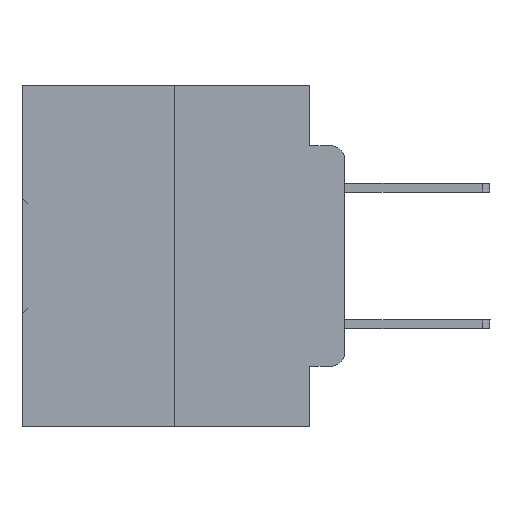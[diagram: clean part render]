
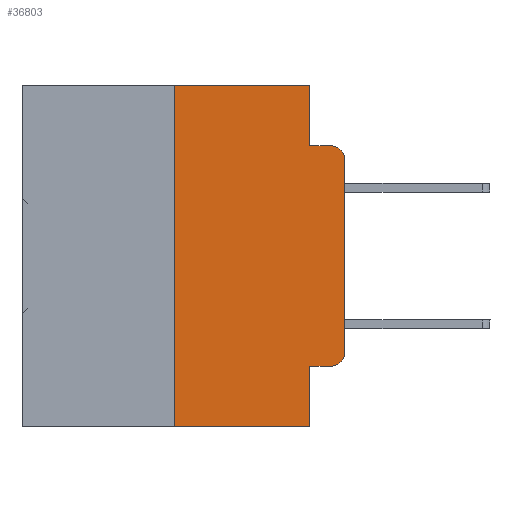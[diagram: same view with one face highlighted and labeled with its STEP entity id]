
A CAD part, left-side view. The second image highlights one B-rep face of the part: STEP entity #36803.
In plain terms, the highlighted planar face has unit normal (-1, 0, 0).
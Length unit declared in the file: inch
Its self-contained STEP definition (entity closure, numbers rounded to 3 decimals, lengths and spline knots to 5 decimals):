
#66 = CARTESIAN_POINT ( 'NONE',  ( 0., 0.02, -0.3915 ) ) ;
#750 = EDGE_CURVE ( 'NONE', #13123, #33339, #28263, .T. ) ;
#777 = VERTEX_POINT ( 'NONE', #26204 ) ;
#805 = ORIENTED_EDGE ( 'NONE', *, *, #27159, .T. ) ;
#1136 = AXIS2_PLACEMENT_3D ( 'NONE', #28376, #11016, #31248 ) ;
#1469 = CARTESIAN_POINT ( 'NONE',  ( 0., 0.051, -0.4115 ) ) ;
#1773 = CIRCLE ( 'NONE', #6889, 0.02 ) ;
#2341 = EDGE_CURVE ( 'NONE', #9298, #10730, #1773, .T. ) ;
#2383 = LINE ( 'NONE', #35653, #30519 ) ;
#2748 = CARTESIAN_POINT ( 'NONE',  ( 0., 0.02, -0.0885 ) ) ;
#4278 = CARTESIAN_POINT ( 'NONE',  ( 0., 0.051, 0. ) ) ;
#4859 = DIRECTION ( 'NONE',  ( 0., 0., 1. ) ) ;
#4932 = ORIENTED_EDGE ( 'NONE', *, *, #24605, .T. ) ;
#5225 = EDGE_CURVE ( 'NONE', #13123, #777, #28075, .T. ) ;
#6889 = AXIS2_PLACEMENT_3D ( 'NONE', #66, #22908, #25892 ) ;
#7152 = DIRECTION ( 'NONE',  ( 0., 0., -1. ) ) ;
#7493 = VECTOR ( 'NONE', #14813, 39.37008 ) ;
#8100 = DIRECTION ( 'NONE',  ( 0., -1., 0. ) ) ;
#8222 = ORIENTED_EDGE ( 'NONE', *, *, #34606, .F. ) ;
#9298 = VERTEX_POINT ( 'NONE', #29091 ) ;
#9443 = EDGE_LOOP ( 'NONE', ( #16734, #4932, #8222, #20383, #10666, #20608, #20315, #22162, #805, #31760 ) ) ;
#10469 = AXIS2_PLACEMENT_3D ( 'NONE', #25110, #33506, #22584 ) ;
#10666 = ORIENTED_EDGE ( 'NONE', *, *, #34669, .F. ) ;
#10730 = VERTEX_POINT ( 'NONE', #23477 ) ;
#10957 = VECTOR ( 'NONE', #28970, 39.37008 ) ;
#11016 = DIRECTION ( 'NONE',  ( 1., 0., 0. ) ) ;
#13123 = VERTEX_POINT ( 'NONE', #31041 ) ;
#13481 = DIRECTION ( 'NONE',  ( 0., -1., 0. ) ) ;
#14813 = DIRECTION ( 'NONE',  ( 0., -1., 0. ) ) ;
#15160 = DIRECTION ( 'NONE',  ( 0., 0., 1. ) ) ;
#15196 = VERTEX_POINT ( 'NONE', #18921 ) ;
#15843 = VECTOR ( 'NONE', #28283, 39.37008 ) ;
#16505 = LINE ( 'NONE', #24801, #18285 ) ;
#16734 = ORIENTED_EDGE ( 'NONE', *, *, #28552, .T. ) ;
#18285 = VECTOR ( 'NONE', #8100, 39.37008 ) ;
#18733 = VECTOR ( 'NONE', #13481, 39.37008 ) ;
#18921 = CARTESIAN_POINT ( 'NONE',  ( 0., 0.051, -0.4115 ) ) ;
#19501 = VERTEX_POINT ( 'NONE', #32627 ) ;
#20314 = CARTESIAN_POINT ( 'NONE',  ( 0., 0.473, -0.5 ) ) ;
#20315 = ORIENTED_EDGE ( 'NONE', *, *, #5225, .T. ) ;
#20383 = ORIENTED_EDGE ( 'NONE', *, *, #35664, .F. ) ;
#20608 = ORIENTED_EDGE ( 'NONE', *, *, #750, .F. ) ;
#21323 = CARTESIAN_POINT ( 'NONE',  ( 0., 0.473, 0. ) ) ;
#21720 = CIRCLE ( 'NONE', #10469, 0.02 ) ;
#22162 = ORIENTED_EDGE ( 'NONE', *, *, #27186, .F. ) ;
#22584 = DIRECTION ( 'NONE',  ( 0., 0., -1. ) ) ;
#22668 = VERTEX_POINT ( 'NONE', #23260 ) ;
#22908 = DIRECTION ( 'NONE',  ( -1., 0., 0. ) ) ;
#23260 = CARTESIAN_POINT ( 'NONE',  ( 0., 0.051, 0. ) ) ;
#23477 = CARTESIAN_POINT ( 'NONE',  ( 0., 0., -0.3915 ) ) ;
#24511 = CARTESIAN_POINT ( 'NONE',  ( 0., 0.25, 0. ) ) ;
#24605 = EDGE_CURVE ( 'NONE', #30196, #31005, #21720, .T. ) ;
#24801 = CARTESIAN_POINT ( 'NONE',  ( 0., 0.051, -0.0885 ) ) ;
#25074 = CARTESIAN_POINT ( 'NONE',  ( 0., 0.25, 0. ) ) ;
#25110 = CARTESIAN_POINT ( 'NONE',  ( 0., 0.02, -0.1085 ) ) ;
#25892 = DIRECTION ( 'NONE',  ( 0., 0., -1. ) ) ;
#26062 = CARTESIAN_POINT ( 'NONE',  ( 0., 0., -0.1085 ) ) ;
#26204 = CARTESIAN_POINT ( 'NONE',  ( 0., 0.051, -0.5 ) ) ;
#27159 = EDGE_CURVE ( 'NONE', #15196, #9298, #27954, .T. ) ;
#27186 = EDGE_CURVE ( 'NONE', #15196, #777, #36423, .T. ) ;
#27954 = LINE ( 'NONE', #1469, #15843 ) ;
#28075 = LINE ( 'NONE', #20314, #7493 ) ;
#28263 = LINE ( 'NONE', #25074, #32244 ) ;
#28283 = DIRECTION ( 'NONE',  ( 0., -1., 0. ) ) ;
#28370 = LINE ( 'NONE', #35002, #10957 ) ;
#28376 = CARTESIAN_POINT ( 'NONE',  ( 0., 0.473, 0. ) ) ;
#28552 = EDGE_CURVE ( 'NONE', #10730, #30196, #2383, .T. ) ;
#28813 = VECTOR ( 'NONE', #7152, 39.37008 ) ;
#28970 = DIRECTION ( 'NONE',  ( 0., 0., -1. ) ) ;
#29091 = CARTESIAN_POINT ( 'NONE',  ( 0., 0.02, -0.4115 ) ) ;
#30075 = FACE_OUTER_BOUND ( 'NONE', #9443, .T. ) ;
#30196 = VERTEX_POINT ( 'NONE', #26062 ) ;
#30519 = VECTOR ( 'NONE', #15160, 39.37008 ) ;
#31005 = VERTEX_POINT ( 'NONE', #2748 ) ;
#31041 = CARTESIAN_POINT ( 'NONE',  ( 0., 0.25, -0.5 ) ) ;
#31131 = PLANE ( 'NONE',  #1136 ) ;
#31248 = DIRECTION ( 'NONE',  ( 0., 0., -1. ) ) ;
#31760 = ORIENTED_EDGE ( 'NONE', *, *, #2341, .T. ) ;
#32244 = VECTOR ( 'NONE', #4859, 39.37008 ) ;
#32627 = CARTESIAN_POINT ( 'NONE',  ( 0., 0.051, -0.0885 ) ) ;
#33339 = VERTEX_POINT ( 'NONE', #24511 ) ;
#33506 = DIRECTION ( 'NONE',  ( -1., 0., 0. ) ) ;
#34606 = EDGE_CURVE ( 'NONE', #19501, #31005, #16505, .T. ) ;
#34669 = EDGE_CURVE ( 'NONE', #33339, #22668, #35709, .T. ) ;
#35002 = CARTESIAN_POINT ( 'NONE',  ( 0., 0.051, 0. ) ) ;
#35653 = CARTESIAN_POINT ( 'NONE',  ( 0., 0., 0. ) ) ;
#35664 = EDGE_CURVE ( 'NONE', #22668, #19501, #28370, .T. ) ;
#35709 = LINE ( 'NONE', #21323, #18733 ) ;
#36423 = LINE ( 'NONE', #4278, #28813 ) ;
#36803 = ADVANCED_FACE ( 'NONE', ( #30075 ), #31131, .F. ) ;
